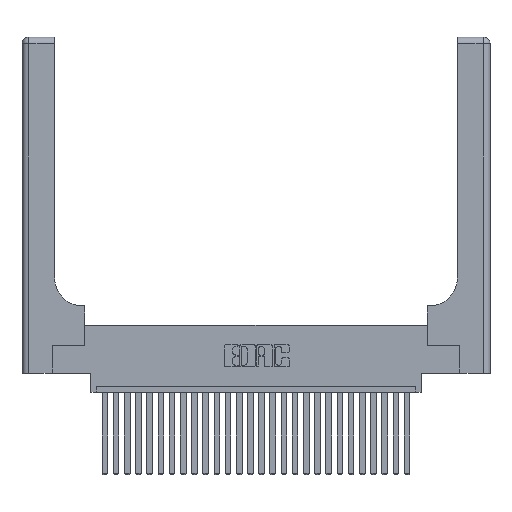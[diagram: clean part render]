
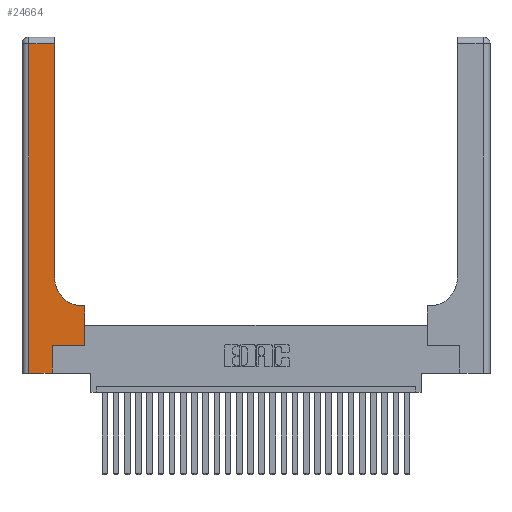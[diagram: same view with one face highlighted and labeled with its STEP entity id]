
A CAD part, top view. The second image highlights one B-rep face of the part: STEP entity #24664.
In plain terms, the highlighted planar face has unit normal (0, 0, 1).
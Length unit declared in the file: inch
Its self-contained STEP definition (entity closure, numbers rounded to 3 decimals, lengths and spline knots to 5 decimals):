
#128 = ORIENTED_EDGE ( 'NONE', *, *, #10468, .T. ) ;
#453 = EDGE_CURVE ( 'NONE', #4695, #22085, #24706, .T. ) ;
#640 = LINE ( 'NONE', #25648, #17278 ) ;
#2120 = VECTOR ( 'NONE', #13168, 39.37008 ) ;
#2160 = PLANE ( 'NONE',  #19441 ) ;
#2533 = ORIENTED_EDGE ( 'NONE', *, *, #27768, .T. ) ;
#3660 = DIRECTION ( 'NONE',  ( 0., 1., 0. ) ) ;
#3965 = VECTOR ( 'NONE', #14773, 39.37008 ) ;
#4362 = DIRECTION ( 'NONE',  ( -1., 0., 0. ) ) ;
#4695 = VERTEX_POINT ( 'NONE', #10602 ) ;
#5412 = ORIENTED_EDGE ( 'NONE', *, *, #27627, .T. ) ;
#5471 = CARTESIAN_POINT ( 'NONE',  ( 0.06, 0., 0.37 ) ) ;
#5752 = CARTESIAN_POINT ( 'NONE',  ( 0.5415, 0.6, 0.37 ) ) ;
#5989 = LINE ( 'NONE', #17034, #3965 ) ;
#6201 = EDGE_CURVE ( 'NONE', #23357, #13725, #640, .T. ) ;
#6915 = LINE ( 'NONE', #27276, #22183 ) ;
#7848 = AXIS2_PLACEMENT_3D ( 'NONE', #11379, #26550, #16110 ) ;
#7875 = LINE ( 'NONE', #8839, #2120 ) ;
#7979 = FACE_OUTER_BOUND ( 'NONE', #13117, .T. ) ;
#8349 = EDGE_CURVE ( 'NONE', #22085, #26145, #24581, .T. ) ;
#8839 = CARTESIAN_POINT ( 'NONE',  ( 0., 2.94, 0.37 ) ) ;
#10468 = EDGE_CURVE ( 'NONE', #13725, #17488, #25354, .T. ) ;
#10602 = CARTESIAN_POINT ( 'NONE',  ( 0.5585, 0.6, 0.37 ) ) ;
#10702 = DIRECTION ( 'NONE',  ( 0., 0., -1. ) ) ;
#11059 = EDGE_CURVE ( 'NONE', #11287, #23357, #5989, .T. ) ;
#11287 = VERTEX_POINT ( 'NONE', #5471 ) ;
#11379 = CARTESIAN_POINT ( 'NONE',  ( 0.5415, 0.85, 0.37 ) ) ;
#11521 = CARTESIAN_POINT ( 'NONE',  ( 0.2915, 0.85, 0.37 ) ) ;
#11565 = ORIENTED_EDGE ( 'NONE', *, *, #14377, .T. ) ;
#11681 = VERTEX_POINT ( 'NONE', #21850 ) ;
#11834 = VECTOR ( 'NONE', #3660, 39.37008 ) ;
#12601 = CARTESIAN_POINT ( 'NONE',  ( 0.269, 0., 0.37 ) ) ;
#13117 = EDGE_LOOP ( 'NONE', ( #21279, #11565, #5412, #14092, #26423, #128, #2533, #16014, #24558 ) ) ;
#13168 = DIRECTION ( 'NONE',  ( -1., 0., 0. ) ) ;
#13198 = CARTESIAN_POINT ( 'NONE',  ( 0.06, 2.94, 0.37 ) ) ;
#13725 = VERTEX_POINT ( 'NONE', #21363 ) ;
#14092 = ORIENTED_EDGE ( 'NONE', *, *, #11059, .T. ) ;
#14377 = EDGE_CURVE ( 'NONE', #11681, #22924, #7875, .T. ) ;
#14773 = DIRECTION ( 'NONE',  ( 1., 0., 0. ) ) ;
#16014 = ORIENTED_EDGE ( 'NONE', *, *, #453, .T. ) ;
#16110 = DIRECTION ( 'NONE',  ( 1., 0., 0. ) ) ;
#17034 = CARTESIAN_POINT ( 'NONE',  ( 0., 0., 0.37 ) ) ;
#17278 = VECTOR ( 'NONE', #26433, 39.37008 ) ;
#17488 = VERTEX_POINT ( 'NONE', #26882 ) ;
#17645 = VECTOR ( 'NONE', #27172, 39.37008 ) ;
#18976 = CARTESIAN_POINT ( 'NONE',  ( 0.269, 0.25, 0.37 ) ) ;
#19441 = AXIS2_PLACEMENT_3D ( 'NONE', #27950, #10702, #4362 ) ;
#19569 = CARTESIAN_POINT ( 'NONE',  ( 0.2915, 0.6, 0.37 ) ) ;
#20437 = CARTESIAN_POINT ( 'NONE',  ( 0.06, 3., 0.37 ) ) ;
#21279 = ORIENTED_EDGE ( 'NONE', *, *, #24409, .T. ) ;
#21363 = CARTESIAN_POINT ( 'NONE',  ( 0.269, 0.25, 0.37 ) ) ;
#21850 = CARTESIAN_POINT ( 'NONE',  ( 0.2915, 2.94, 0.37 ) ) ;
#22085 = VERTEX_POINT ( 'NONE', #5752 ) ;
#22183 = VECTOR ( 'NONE', #22720, 39.37008 ) ;
#22695 = LINE ( 'NONE', #23081, #11834 ) ;
#22720 = DIRECTION ( 'NONE',  ( 0., 1., 0. ) ) ;
#22924 = VERTEX_POINT ( 'NONE', #13198 ) ;
#23081 = CARTESIAN_POINT ( 'NONE',  ( 0.5585, 0.25, 0.37 ) ) ;
#23342 = DIRECTION ( 'NONE',  ( 1., 0., 0. ) ) ;
#23357 = VERTEX_POINT ( 'NONE', #12601 ) ;
#24051 = VECTOR ( 'NONE', #26014, 39.37008 ) ;
#24409 = EDGE_CURVE ( 'NONE', #26145, #11681, #6915, .T. ) ;
#24558 = ORIENTED_EDGE ( 'NONE', *, *, #8349, .T. ) ;
#24581 = CIRCLE ( 'NONE', #7848, 0.25 ) ;
#24664 = ADVANCED_FACE ( 'NONE', ( #7979 ), #2160, .F. ) ;
#24706 = LINE ( 'NONE', #19569, #24051 ) ;
#25354 = LINE ( 'NONE', #18976, #25681 ) ;
#25648 = CARTESIAN_POINT ( 'NONE',  ( 0.269, 0., 0.37 ) ) ;
#25681 = VECTOR ( 'NONE', #23342, 39.37008 ) ;
#26014 = DIRECTION ( 'NONE',  ( -1., 0., 0. ) ) ;
#26145 = VERTEX_POINT ( 'NONE', #11521 ) ;
#26423 = ORIENTED_EDGE ( 'NONE', *, *, #6201, .T. ) ;
#26433 = DIRECTION ( 'NONE',  ( 0., 1., 0. ) ) ;
#26550 = DIRECTION ( 'NONE',  ( 0., 0., -1. ) ) ;
#26882 = CARTESIAN_POINT ( 'NONE',  ( 0.5585, 0.25, 0.37 ) ) ;
#27172 = DIRECTION ( 'NONE',  ( 0., -1., 0. ) ) ;
#27276 = CARTESIAN_POINT ( 'NONE',  ( 0.2915, 3., 0.37 ) ) ;
#27467 = LINE ( 'NONE', #20437, #17645 ) ;
#27627 = EDGE_CURVE ( 'NONE', #22924, #11287, #27467, .T. ) ;
#27768 = EDGE_CURVE ( 'NONE', #17488, #4695, #22695, .T. ) ;
#27950 = CARTESIAN_POINT ( 'NONE',  ( 0., 3., 0.37 ) ) ;
